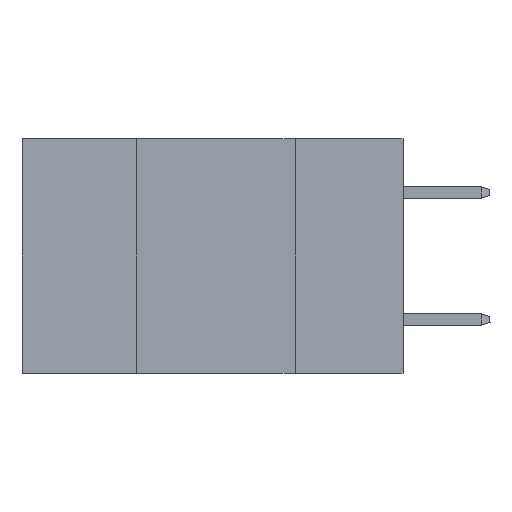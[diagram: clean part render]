
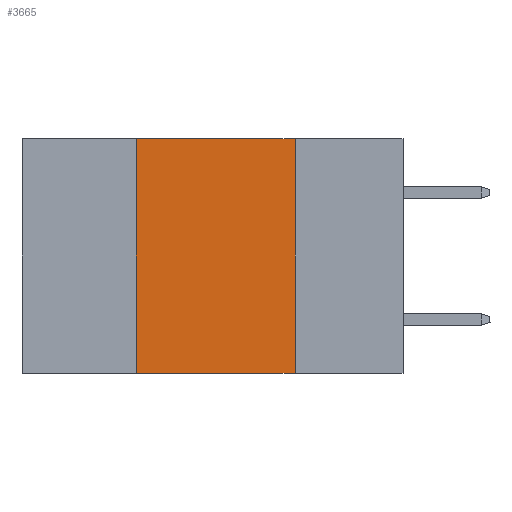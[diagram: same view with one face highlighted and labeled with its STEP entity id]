
A CAD part, left-side view. The second image highlights one B-rep face of the part: STEP entity #3665.
In plain terms, the highlighted planar face has unit normal (-1, 0, 0).
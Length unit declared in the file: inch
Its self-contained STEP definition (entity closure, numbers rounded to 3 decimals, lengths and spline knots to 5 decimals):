
#31 = ORIENTED_EDGE ( 'NONE', *, *, #10578, .F. ) ;
#398 = EDGE_CURVE ( 'NONE', #13305, #11708, #11756, .T. ) ;
#1108 = VERTEX_POINT ( 'NONE', #3160 ) ;
#1113 = DIRECTION ( 'NONE',  ( 1., 0., 0. ) ) ;
#1231 = VERTEX_POINT ( 'NONE', #6473 ) ;
#1261 = VECTOR ( 'NONE', #2248, 39.37008 ) ;
#1648 = DIRECTION ( 'NONE',  ( 0., 0., -1. ) ) ;
#1856 = LINE ( 'NONE', #5122, #10414 ) ;
#2248 = DIRECTION ( 'NONE',  ( 0., -1., 0. ) ) ;
#2508 = VECTOR ( 'NONE', #2950, 39.37008 ) ;
#2950 = DIRECTION ( 'NONE',  ( 0., 0., 1. ) ) ;
#3160 = CARTESIAN_POINT ( 'NONE',  ( 0., 0.42, 0. ) ) ;
#3665 = ADVANCED_FACE ( 'NONE', ( #7418 ), #6386, .F. ) ;
#4013 = AXIS2_PLACEMENT_3D ( 'NONE', #10621, #1113, #5354 ) ;
#4984 = EDGE_CURVE ( 'NONE', #13305, #1108, #12441, .T. ) ;
#5122 = CARTESIAN_POINT ( 'NONE',  ( 0., 0.17, 0. ) ) ;
#5354 = DIRECTION ( 'NONE',  ( 0., 0., -1. ) ) ;
#5378 = ORIENTED_EDGE ( 'NONE', *, *, #6564, .F. ) ;
#5560 = DIRECTION ( 'NONE',  ( 0., -1., 0. ) ) ;
#6054 = ORIENTED_EDGE ( 'NONE', *, *, #398, .T. ) ;
#6337 = CARTESIAN_POINT ( 'NONE',  ( 0., 0.17, -0.37 ) ) ;
#6386 = PLANE ( 'NONE',  #4013 ) ;
#6473 = CARTESIAN_POINT ( 'NONE',  ( 0., 0.17, 0. ) ) ;
#6564 = EDGE_CURVE ( 'NONE', #1108, #1231, #9845, .T. ) ;
#7418 = FACE_OUTER_BOUND ( 'NONE', #12754, .T. ) ;
#8467 = CARTESIAN_POINT ( 'NONE',  ( 0., 0.42, 0. ) ) ;
#9312 = CARTESIAN_POINT ( 'NONE',  ( 0., 0.6, -0.37 ) ) ;
#9845 = LINE ( 'NONE', #12020, #12731 ) ;
#10405 = ORIENTED_EDGE ( 'NONE', *, *, #4984, .F. ) ;
#10414 = VECTOR ( 'NONE', #1648, 39.37008 ) ;
#10578 = EDGE_CURVE ( 'NONE', #1231, #11708, #1856, .T. ) ;
#10621 = CARTESIAN_POINT ( 'NONE',  ( 0., 0.6, 0. ) ) ;
#11708 = VERTEX_POINT ( 'NONE', #6337 ) ;
#11756 = LINE ( 'NONE', #9312, #1261 ) ;
#12020 = CARTESIAN_POINT ( 'NONE',  ( 0., 0.6, 0. ) ) ;
#12441 = LINE ( 'NONE', #8467, #2508 ) ;
#12731 = VECTOR ( 'NONE', #5560, 39.37008 ) ;
#12754 = EDGE_LOOP ( 'NONE', ( #31, #5378, #10405, #6054 ) ) ;
#13305 = VERTEX_POINT ( 'NONE', #13412 ) ;
#13412 = CARTESIAN_POINT ( 'NONE',  ( 0., 0.42, -0.37 ) ) ;
